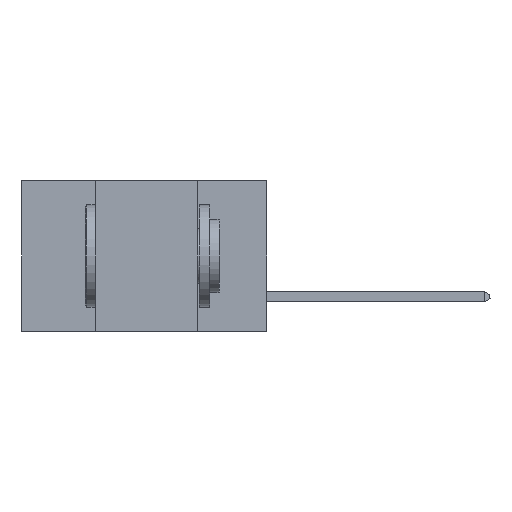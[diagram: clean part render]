
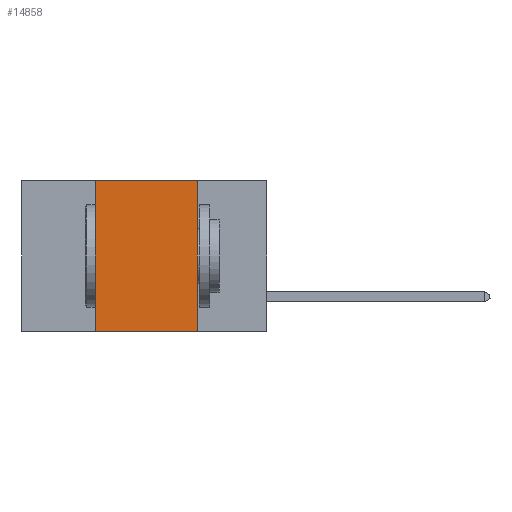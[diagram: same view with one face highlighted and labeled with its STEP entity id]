
A CAD part, left-side view. The second image highlights one B-rep face of the part: STEP entity #14858.
In plain terms, the highlighted planar face has unit normal (-1, 0, 0).
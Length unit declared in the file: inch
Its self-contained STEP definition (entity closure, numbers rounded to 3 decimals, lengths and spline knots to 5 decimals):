
#91 = CARTESIAN_POINT ( 'NONE',  ( 0., 0.6, 0. ) ) ;
#3953 = LINE ( 'NONE', #35361, #14168 ) ;
#5172 = DIRECTION ( 'NONE',  ( 0., 0., 1. ) ) ;
#5466 = CARTESIAN_POINT ( 'NONE',  ( 0., 0.6, 0. ) ) ;
#8084 = DIRECTION ( 'NONE',  ( 0., 0., -1. ) ) ;
#9205 = DIRECTION ( 'NONE',  ( 0., -1., 0. ) ) ;
#10112 = EDGE_CURVE ( 'NONE', #35224, #33675, #26901, .T. ) ;
#11151 = ORIENTED_EDGE ( 'NONE', *, *, #10112, .F. ) ;
#11849 = LINE ( 'NONE', #12219, #32859 ) ;
#12219 = CARTESIAN_POINT ( 'NONE',  ( 0., 0.6, -0.37 ) ) ;
#13706 = ORIENTED_EDGE ( 'NONE', *, *, #25996, .T. ) ;
#14034 = PLANE ( 'NONE',  #19048 ) ;
#14168 = VECTOR ( 'NONE', #17927, 39.37008 ) ;
#14858 = ADVANCED_FACE ( 'NONE', ( #33524 ), #14034, .F. ) ;
#14904 = LINE ( 'NONE', #91, #26586 ) ;
#15295 = CARTESIAN_POINT ( 'NONE',  ( 0., 0.17, 0. ) ) ;
#16771 = DIRECTION ( 'NONE',  ( 1., 0., 0. ) ) ;
#17927 = DIRECTION ( 'NONE',  ( 0., 0., -1. ) ) ;
#19048 = AXIS2_PLACEMENT_3D ( 'NONE', #5466, #16771, #8084 ) ;
#20239 = EDGE_LOOP ( 'NONE', ( #36181, #26054, #11151, #13706 ) ) ;
#25530 = CARTESIAN_POINT ( 'NONE',  ( 0., 0.42, -0.37 ) ) ;
#25549 = CARTESIAN_POINT ( 'NONE',  ( 0., 0.42, 0. ) ) ;
#25550 = EDGE_CURVE ( 'NONE', #26674, #30081, #3953, .T. ) ;
#25996 = EDGE_CURVE ( 'NONE', #35224, #30081, #11849, .T. ) ;
#26054 = ORIENTED_EDGE ( 'NONE', *, *, #28917, .F. ) ;
#26586 = VECTOR ( 'NONE', #9205, 39.37008 ) ;
#26674 = VERTEX_POINT ( 'NONE', #15295 ) ;
#26901 = LINE ( 'NONE', #31646, #28776 ) ;
#28776 = VECTOR ( 'NONE', #5172, 39.37008 ) ;
#28917 = EDGE_CURVE ( 'NONE', #33675, #26674, #14904, .T. ) ;
#29837 = DIRECTION ( 'NONE',  ( 0., -1., 0. ) ) ;
#30081 = VERTEX_POINT ( 'NONE', #38283 ) ;
#31646 = CARTESIAN_POINT ( 'NONE',  ( 0., 0.42, 0. ) ) ;
#32859 = VECTOR ( 'NONE', #29837, 39.37008 ) ;
#33524 = FACE_OUTER_BOUND ( 'NONE', #20239, .T. ) ;
#33675 = VERTEX_POINT ( 'NONE', #25549 ) ;
#35224 = VERTEX_POINT ( 'NONE', #25530 ) ;
#35361 = CARTESIAN_POINT ( 'NONE',  ( 0., 0.17, 0. ) ) ;
#36181 = ORIENTED_EDGE ( 'NONE', *, *, #25550, .F. ) ;
#38283 = CARTESIAN_POINT ( 'NONE',  ( 0., 0.17, -0.37 ) ) ;
